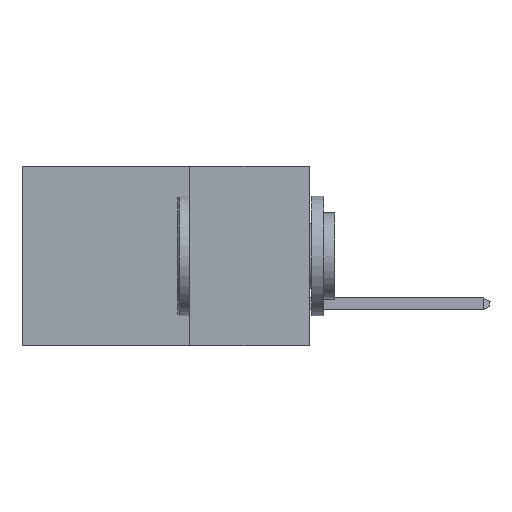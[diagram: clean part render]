
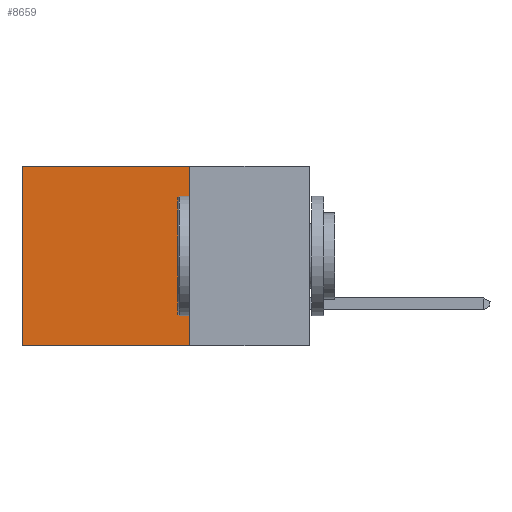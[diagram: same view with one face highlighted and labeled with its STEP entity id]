
A CAD part, left-side view. The second image highlights one B-rep face of the part: STEP entity #8659.
In plain terms, the highlighted planar face has unit normal (-1, 0, 0).
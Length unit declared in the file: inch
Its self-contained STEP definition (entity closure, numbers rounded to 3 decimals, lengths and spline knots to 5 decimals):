
#367 = VECTOR ( 'NONE', #2082, 39.37008 ) ;
#750 = ORIENTED_EDGE ( 'NONE', *, *, #4802, .T. ) ;
#993 = ORIENTED_EDGE ( 'NONE', *, *, #7153, .T. ) ;
#1393 = CARTESIAN_POINT ( 'NONE',  ( 0.2875, 0.25, -0.375 ) ) ;
#1527 = LINE ( 'NONE', #4443, #4907 ) ;
#1853 = LINE ( 'NONE', #7339, #5901 ) ;
#2082 = DIRECTION ( 'NONE',  ( 0., 0., -1. ) ) ;
#2123 = DIRECTION ( 'NONE',  ( 0., 1., 0. ) ) ;
#2982 = VERTEX_POINT ( 'NONE', #3058 ) ;
#3016 = CARTESIAN_POINT ( 'NONE',  ( 0.2875, 0.25, 0. ) ) ;
#3058 = CARTESIAN_POINT ( 'NONE',  ( 0.2875, 0.6, -0.375 ) ) ;
#3504 = EDGE_CURVE ( 'NONE', #5477, #6354, #7867, .T. ) ;
#3668 = AXIS2_PLACEMENT_3D ( 'NONE', #8465, #8227, #4046 ) ;
#4046 = DIRECTION ( 'NONE',  ( 0., 0., -1. ) ) ;
#4104 = CARTESIAN_POINT ( 'NONE',  ( 0.2875, 0.6, 0. ) ) ;
#4246 = VECTOR ( 'NONE', #2123, 39.37008 ) ;
#4414 = DIRECTION ( 'NONE',  ( 0., 0., -1. ) ) ;
#4443 = CARTESIAN_POINT ( 'NONE',  ( 0.2875, 0.6, -0.375 ) ) ;
#4802 = EDGE_CURVE ( 'NONE', #6407, #2982, #1527, .T. ) ;
#4907 = VECTOR ( 'NONE', #4414, 39.37008 ) ;
#4908 = CARTESIAN_POINT ( 'NONE',  ( 0.2875, 0.25, -0.375 ) ) ;
#5001 = FACE_OUTER_BOUND ( 'NONE', #6390, .T. ) ;
#5166 = ORIENTED_EDGE ( 'NONE', *, *, #8118, .F. ) ;
#5477 = VERTEX_POINT ( 'NONE', #3016 ) ;
#5901 = VECTOR ( 'NONE', #7967, 39.37008 ) ;
#6354 = VERTEX_POINT ( 'NONE', #8711 ) ;
#6390 = EDGE_LOOP ( 'NONE', ( #750, #5166, #8865, #993 ) ) ;
#6407 = VERTEX_POINT ( 'NONE', #4104 ) ;
#7153 = EDGE_CURVE ( 'NONE', #5477, #6407, #1853, .T. ) ;
#7339 = CARTESIAN_POINT ( 'NONE',  ( 0.2875, 0.25, 0. ) ) ;
#7867 = LINE ( 'NONE', #1393, #367 ) ;
#7953 = LINE ( 'NONE', #4908, #4246 ) ;
#7967 = DIRECTION ( 'NONE',  ( 0., 1., 0. ) ) ;
#8118 = EDGE_CURVE ( 'NONE', #6354, #2982, #7953, .T. ) ;
#8227 = DIRECTION ( 'NONE',  ( 1., 0., 0. ) ) ;
#8465 = CARTESIAN_POINT ( 'NONE',  ( 0.2875, 0.25, -0.375 ) ) ;
#8659 = ADVANCED_FACE ( 'NONE', ( #5001 ), #8944, .F. ) ;
#8711 = CARTESIAN_POINT ( 'NONE',  ( 0.2875, 0.25, -0.375 ) ) ;
#8865 = ORIENTED_EDGE ( 'NONE', *, *, #3504, .F. ) ;
#8944 = PLANE ( 'NONE',  #3668 ) ;
